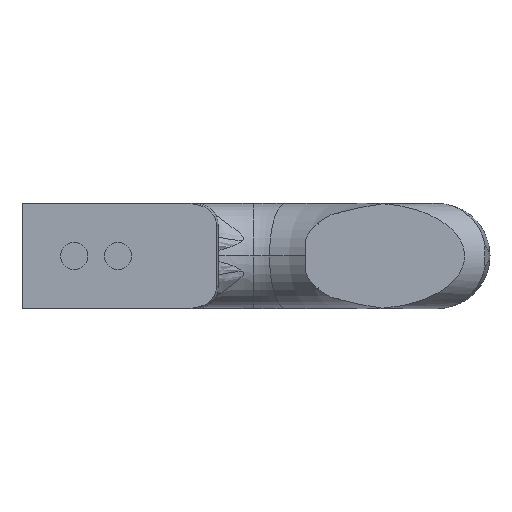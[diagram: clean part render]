
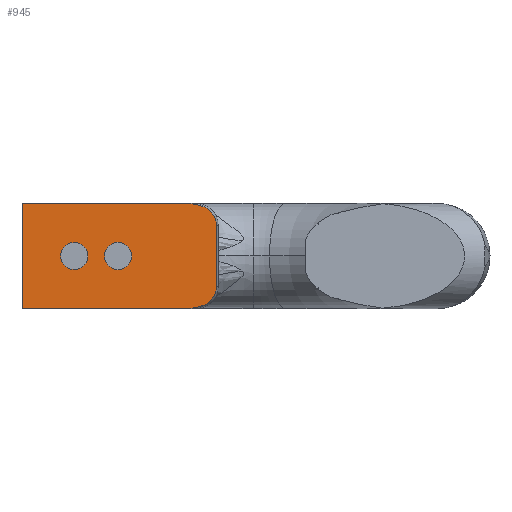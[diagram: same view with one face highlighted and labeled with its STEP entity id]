
A CAD part, left-side view. The second image highlights one B-rep face of the part: STEP entity #945.
In plain terms, the highlighted planar face has unit normal (-1, 0, 0).
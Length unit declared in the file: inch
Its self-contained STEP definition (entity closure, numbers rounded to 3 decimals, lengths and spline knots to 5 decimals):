
#57 = CIRCLE ( 'NONE', #2905, 0.12205 ) ;
#63 = CARTESIAN_POINT ( 'NONE',  ( 8.2556, -0.98436, 0. ) ) ;
#159 = ORIENTED_EDGE ( 'NONE', *, *, #2841, .T. ) ;
#171 = VERTEX_POINT ( 'NONE', #1275 ) ;
#198 = FACE_BOUND ( 'NONE', #1893, .T. ) ;
#229 = CARTESIAN_POINT ( 'NONE',  ( 8.2556, -1.10641, 0. ) ) ;
#240 = VERTEX_POINT ( 'NONE', #422 ) ;
#265 = VERTEX_POINT ( 'NONE', #434 ) ;
#282 = CARTESIAN_POINT ( 'NONE',  ( 8.2556, -2.10137, 0.46161 ) ) ;
#308 = CARTESIAN_POINT ( 'NONE',  ( 8.2556, -1.25602, 0. ) ) ;
#361 = DIRECTION ( 'NONE',  ( 0., 1., 0. ) ) ;
#422 = CARTESIAN_POINT ( 'NONE',  ( 8.2556, -2.15109, 0.44083 ) ) ;
#434 = CARTESIAN_POINT ( 'NONE',  ( 8.2556, -2.26111, 0.27559 ) ) ;
#455 = DIRECTION ( 'NONE',  ( 0., 1., 0. ) ) ;
#535 = ORIENTED_EDGE ( 'NONE', *, *, #2799, .T. ) ;
#571 = VECTOR ( 'NONE', #881, 39.37008 ) ;
#588 = DIRECTION ( 'NONE',  ( -1., 0., 0. ) ) ;
#607 = CARTESIAN_POINT ( 'NONE',  ( 8.2556, -3.1632, -0.47244 ) ) ;
#664 = VECTOR ( 'NONE', #2547, 39.37008 ) ;
#684 = VERTEX_POINT ( 'NONE', #2261 ) ;
#717 = CIRCLE ( 'NONE', #784, 0.12205 ) ;
#760 = LINE ( 'NONE', #861, #2888 ) ;
#784 = AXIS2_PLACEMENT_3D ( 'NONE', #1549, #3510, #1821 ) ;
#802 = CIRCLE ( 'NONE', #871, 0.12205 ) ;
#810 = ORIENTED_EDGE ( 'NONE', *, *, #1892, .T. ) ;
#848 = DIRECTION ( 'NONE',  ( 0., 0., 1. ) ) ;
#861 = CARTESIAN_POINT ( 'NONE',  ( 8.2556, -2.26111, -0.27559 ) ) ;
#871 = AXIS2_PLACEMENT_3D ( 'NONE', #1249, #3206, #1526 ) ;
#874 = DIRECTION ( 'NONE',  ( 0., 1., 0. ) ) ;
#876 = CARTESIAN_POINT ( 'NONE',  ( 8.2556, -1.50011, 0. ) ) ;
#881 = DIRECTION ( 'NONE',  ( 0., 0., 1. ) ) ;
#885 = FACE_OUTER_BOUND ( 'NONE', #997, .T. ) ;
#933 = ORIENTED_EDGE ( 'NONE', *, *, #2826, .T. ) ;
#945 = ADVANCED_FACE ( 'NONE', ( #198, #2371, #885 ), #3529, .F. ) ;
#997 = EDGE_LOOP ( 'NONE', ( #535, #2575, #933, #159, #2318, #1468, #2344, #3361 ) ) ;
#1008 = VERTEX_POINT ( 'NONE', #1040 ) ;
#1009 = AXIS2_PLACEMENT_3D ( 'NONE', #63, #2039, #361 ) ;
#1040 = CARTESIAN_POINT ( 'NONE',  ( 8.2556, -1.98535, 0.47244 ) ) ;
#1123 = DIRECTION ( 'NONE',  ( 1., 0., 0. ) ) ;
#1134 = DIRECTION ( 'NONE',  ( -1., 0., 0. ) ) ;
#1147 = CARTESIAN_POINT ( 'NONE',  ( 8.2556, -1.98535, 0.47244 ) ) ;
#1249 = CARTESIAN_POINT ( 'NONE',  ( 8.2556, -1.37807, 0. ) ) ;
#1275 = CARTESIAN_POINT ( 'NONE',  ( 8.2556, -0.51472, -0.47244 ) ) ;
#1338 = EDGE_LOOP ( 'NONE', ( #2197, #2848 ) ) ;
#1403 = CIRCLE ( 'NONE', #2660, 0.17909 ) ;
#1419 = VERTEX_POINT ( 'NONE', #876 ) ;
#1468 = ORIENTED_EDGE ( 'NONE', *, *, #2867, .T. ) ;
#1485 = CIRCLE ( 'NONE', #2849, 0.17909 ) ;
#1526 = DIRECTION ( 'NONE',  ( 0., 1., 0. ) ) ;
#1549 = CARTESIAN_POINT ( 'NONE',  ( 8.2556, -1.37807, 0. ) ) ;
#1557 = AXIS2_PLACEMENT_3D ( 'NONE', #1841, #2387, #455 ) ;
#1562 = EDGE_CURVE ( 'NONE', #2728, #3483, #3205, .T. ) ;
#1593 = VERTEX_POINT ( 'NONE', #2326 ) ;
#1676 = CARTESIAN_POINT ( 'NONE',  ( 8.2556, -2.15109, -0.44083 ) ) ;
#1677 = VERTEX_POINT ( 'NONE', #2343 ) ;
#1688 = CARTESIAN_POINT ( 'NONE',  ( 8.2556, -0.51472, -0.70907 ) ) ;
#1708 = ORIENTED_EDGE ( 'NONE', *, *, #1765, .T. ) ;
#1733 = VERTEX_POINT ( 'NONE', #2057 ) ;
#1765 = EDGE_CURVE ( 'NONE', #1419, #2912, #802, .T. ) ;
#1821 = DIRECTION ( 'NONE',  ( 0., 1., 0. ) ) ;
#1841 = CARTESIAN_POINT ( 'NONE',  ( 8.2556, -5.33922, 2.87623 ) ) ;
#1892 = EDGE_CURVE ( 'NONE', #2912, #1419, #717, .T. ) ;
#1893 = EDGE_LOOP ( 'NONE', ( #1708, #810 ) ) ;
#1925 = CARTESIAN_POINT ( 'NONE',  ( 8.2556, -2.04457, -0.47244 ) ) ;
#1936 = CARTESIAN_POINT ( 'NONE',  ( 8.2556, -1.98535, -0.47244 ) ) ;
#1956 = LINE ( 'NONE', #607, #664 ) ;
#2039 = DIRECTION ( 'NONE',  ( 1., 0., 0. ) ) ;
#2057 = CARTESIAN_POINT ( 'NONE',  ( 8.2556, -0.51472, 0.47244 ) ) ;
#2197 = ORIENTED_EDGE ( 'NONE', *, *, #1562, .T. ) ;
#2232 = LINE ( 'NONE', #2519, #3554 ) ;
#2254 = CARTESIAN_POINT ( 'NONE',  ( 8.2556, -2.08202, 0.27559 ) ) ;
#2261 = CARTESIAN_POINT ( 'NONE',  ( 8.2556, -2.15109, -0.44083 ) ) ;
#2318 = ORIENTED_EDGE ( 'NONE', *, *, #2846, .T. ) ;
#2326 = CARTESIAN_POINT ( 'NONE',  ( 8.2556, -1.98535, -0.47244 ) ) ;
#2343 = CARTESIAN_POINT ( 'NONE',  ( 8.2556, -2.26111, -0.27559 ) ) ;
#2344 = ORIENTED_EDGE ( 'NONE', *, *, #2896, .F. ) ;
#2371 = FACE_BOUND ( 'NONE', #1338, .T. ) ;
#2387 = DIRECTION ( 'NONE',  ( 1., 0., 0. ) ) ;
#2519 = CARTESIAN_POINT ( 'NONE',  ( 8.2556, -2.3896, 0.47244 ) ) ;
#2529 = DIRECTION ( 'NONE',  ( 0., 1., 0. ) ) ;
#2547 = DIRECTION ( 'NONE',  ( 0., 1., 0. ) ) ;
#2575 = ORIENTED_EDGE ( 'NONE', *, *, #2821, .T. ) ;
#2660 = AXIS2_PLACEMENT_3D ( 'NONE', #2254, #588, #2529 ) ;
#2717 =( BOUNDED_CURVE ( )  B_SPLINE_CURVE ( 3, ( #1936, #1925, #3363, #1676 ),
 .UNSPECIFIED., .F., .F. ) 
 B_SPLINE_CURVE_WITH_KNOTS ( ( 4, 4 ),
 ( 1.5708, 2.14542 ),
 .UNSPECIFIED. ) 
 CURVE ( )  GEOMETRIC_REPRESENTATION_ITEM ( )  RATIONAL_B_SPLINE_CURVE ( ( 1., 0.973, 0.973, 1. ) ) 
 REPRESENTATION_ITEM ( '' )  );
#2728 = VERTEX_POINT ( 'NONE', #229 ) ;
#2775 = EDGE_CURVE ( 'NONE', #3483, #2728, #57, .T. ) ;
#2777 =( BOUNDED_CURVE ( )  B_SPLINE_CURVE ( 3, ( #3655, #282, #2814, #1147 ),
 .UNSPECIFIED., .F., .F. ) 
 B_SPLINE_CURVE_WITH_KNOTS ( ( 4, 4 ),
 ( 4.13777, 4.71239 ),
 .UNSPECIFIED. ) 
 CURVE ( )  GEOMETRIC_REPRESENTATION_ITEM ( )  RATIONAL_B_SPLINE_CURVE ( ( 1., 0.973, 0.973, 1. ) ) 
 REPRESENTATION_ITEM ( '' )  );
#2787 = CARTESIAN_POINT ( 'NONE',  ( 8.2556, -0.98436, 0. ) ) ;
#2799 = EDGE_CURVE ( 'NONE', #1593, #684, #2717, .T. ) ;
#2803 = CARTESIAN_POINT ( 'NONE',  ( 8.2556, -2.08202, -0.27559 ) ) ;
#2814 = CARTESIAN_POINT ( 'NONE',  ( 8.2556, -2.04457, 0.47244 ) ) ;
#2821 = EDGE_CURVE ( 'NONE', #684, #1677, #1485, .T. ) ;
#2826 = EDGE_CURVE ( 'NONE', #1677, #265, #760, .T. ) ;
#2841 = EDGE_CURVE ( 'NONE', #265, #240, #1403, .T. ) ;
#2846 = EDGE_CURVE ( 'NONE', #240, #1008, #2777, .T. ) ;
#2848 = ORIENTED_EDGE ( 'NONE', *, *, #2775, .T. ) ;
#2849 = AXIS2_PLACEMENT_3D ( 'NONE', #2803, #1134, #3094 ) ;
#2867 = EDGE_CURVE ( 'NONE', #1008, #1733, #2232, .T. ) ;
#2888 = VECTOR ( 'NONE', #848, 39.37008 ) ;
#2896 = EDGE_CURVE ( 'NONE', #171, #1733, #3640, .T. ) ;
#2904 = EDGE_CURVE ( 'NONE', #1593, #171, #1956, .T. ) ;
#2905 = AXIS2_PLACEMENT_3D ( 'NONE', #2787, #1123, #3081 ) ;
#2912 = VERTEX_POINT ( 'NONE', #308 ) ;
#3081 = DIRECTION ( 'NONE',  ( 0., 1., 0. ) ) ;
#3094 = DIRECTION ( 'NONE',  ( 0., 1., 0. ) ) ;
#3205 = CIRCLE ( 'NONE', #1009, 0.12205 ) ;
#3206 = DIRECTION ( 'NONE',  ( 1., 0., 0. ) ) ;
#3361 = ORIENTED_EDGE ( 'NONE', *, *, #2904, .F. ) ;
#3363 = CARTESIAN_POINT ( 'NONE',  ( 8.2556, -2.10137, -0.46161 ) ) ;
#3483 = VERTEX_POINT ( 'NONE', #3505 ) ;
#3505 = CARTESIAN_POINT ( 'NONE',  ( 8.2556, -0.86232, 0. ) ) ;
#3510 = DIRECTION ( 'NONE',  ( 1., 0., 0. ) ) ;
#3529 = PLANE ( 'NONE',  #1557 ) ;
#3554 = VECTOR ( 'NONE', #874, 39.37008 ) ;
#3640 = LINE ( 'NONE', #1688, #571 ) ;
#3655 = CARTESIAN_POINT ( 'NONE',  ( 8.2556, -2.15109, 0.44083 ) ) ;
